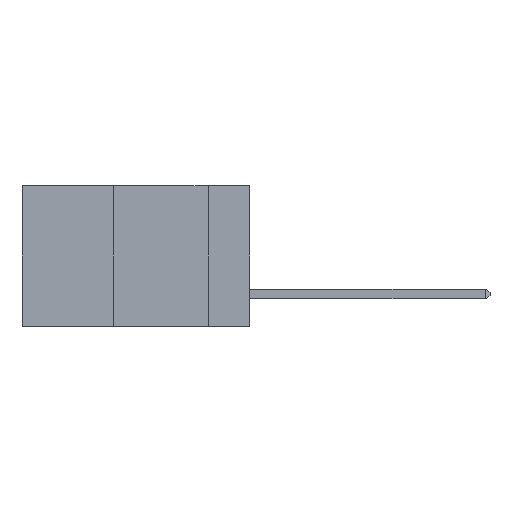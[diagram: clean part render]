
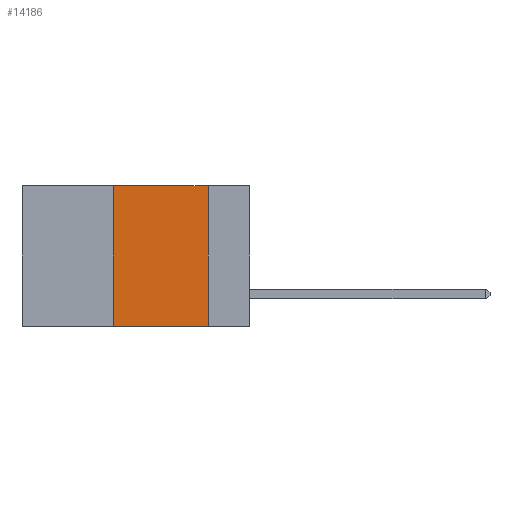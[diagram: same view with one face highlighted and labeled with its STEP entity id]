
A CAD part, left-side view. The second image highlights one B-rep face of the part: STEP entity #14186.
In plain terms, the highlighted planar face has unit normal (-1, 0, 0).
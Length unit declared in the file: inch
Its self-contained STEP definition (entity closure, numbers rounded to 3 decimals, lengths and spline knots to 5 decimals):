
#260 = EDGE_CURVE ( 'NONE', #9420, #14748, #11867, .T. ) ;
#1871 = PLANE ( 'NONE',  #18683 ) ;
#3011 = CARTESIAN_POINT ( 'NONE',  ( 0., 0.36, 0. ) ) ;
#3241 = CARTESIAN_POINT ( 'NONE',  ( 0., 0.11, -0.37 ) ) ;
#3336 = VECTOR ( 'NONE', #11505, 39.37008 ) ;
#4752 = EDGE_CURVE ( 'NONE', #9420, #19886, #8857, .T. ) ;
#5828 = LINE ( 'NONE', #13380, #13806 ) ;
#5899 = EDGE_CURVE ( 'NONE', #17694, #14748, #5828, .T. ) ;
#6598 = EDGE_LOOP ( 'NONE', ( #12681, #17683, #9256, #13742 ) ) ;
#6720 = CARTESIAN_POINT ( 'NONE',  ( 0., 0.36, 0. ) ) ;
#7268 = EDGE_CURVE ( 'NONE', #19886, #17694, #18206, .T. ) ;
#7823 = CARTESIAN_POINT ( 'NONE',  ( 0., 0.36, -0.37 ) ) ;
#8716 = DIRECTION ( 'NONE',  ( 0., 0., -1. ) ) ;
#8725 = VECTOR ( 'NONE', #17076, 39.37008 ) ;
#8857 = LINE ( 'NONE', #6720, #17813 ) ;
#9256 = ORIENTED_EDGE ( 'NONE', *, *, #4752, .F. ) ;
#9420 = VERTEX_POINT ( 'NONE', #7823 ) ;
#11505 = DIRECTION ( 'NONE',  ( 0., -1., 0. ) ) ;
#11867 = LINE ( 'NONE', #16690, #3336 ) ;
#12681 = ORIENTED_EDGE ( 'NONE', *, *, #5899, .F. ) ;
#13380 = CARTESIAN_POINT ( 'NONE',  ( 0., 0.11, 0. ) ) ;
#13742 = ORIENTED_EDGE ( 'NONE', *, *, #260, .T. ) ;
#13806 = VECTOR ( 'NONE', #18440, 39.37008 ) ;
#14186 = ADVANCED_FACE ( 'NONE', ( #14462 ), #1871, .F. ) ;
#14462 = FACE_OUTER_BOUND ( 'NONE', #6598, .T. ) ;
#14748 = VERTEX_POINT ( 'NONE', #3241 ) ;
#16690 = CARTESIAN_POINT ( 'NONE',  ( 0., 0.6, -0.37 ) ) ;
#16880 = DIRECTION ( 'NONE',  ( 0., 0., 1. ) ) ;
#17076 = DIRECTION ( 'NONE',  ( 0., -1., 0. ) ) ;
#17123 = CARTESIAN_POINT ( 'NONE',  ( 0., 0.6, 0. ) ) ;
#17683 = ORIENTED_EDGE ( 'NONE', *, *, #7268, .F. ) ;
#17694 = VERTEX_POINT ( 'NONE', #19437 ) ;
#17813 = VECTOR ( 'NONE', #16880, 39.37008 ) ;
#18206 = LINE ( 'NONE', #18757, #8725 ) ;
#18440 = DIRECTION ( 'NONE',  ( 0., 0., -1. ) ) ;
#18683 = AXIS2_PLACEMENT_3D ( 'NONE', #17123, #18801, #8716 ) ;
#18757 = CARTESIAN_POINT ( 'NONE',  ( 0., 0.6, 0. ) ) ;
#18801 = DIRECTION ( 'NONE',  ( 1., 0., 0. ) ) ;
#19437 = CARTESIAN_POINT ( 'NONE',  ( 0., 0.11, 0. ) ) ;
#19886 = VERTEX_POINT ( 'NONE', #3011 ) ;
